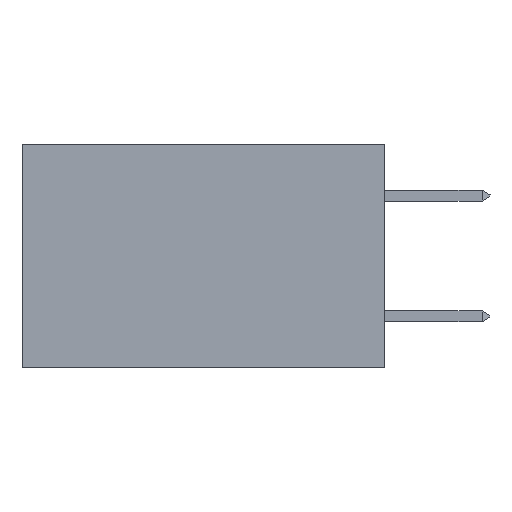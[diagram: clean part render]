
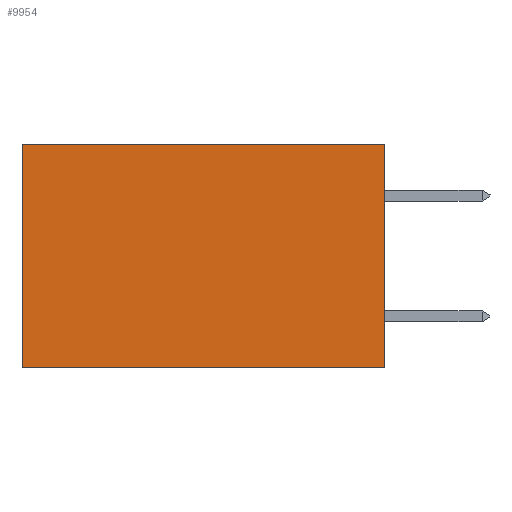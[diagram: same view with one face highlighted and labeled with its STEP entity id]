
A CAD part, left-side view. The second image highlights one B-rep face of the part: STEP entity #9954.
In plain terms, the highlighted planar face has unit normal (-1, 0, 0).
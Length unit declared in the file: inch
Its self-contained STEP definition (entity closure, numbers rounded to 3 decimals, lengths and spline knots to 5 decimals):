
#1040 = VECTOR ( 'NONE', #24002, 39.37008 ) ;
#1258 = LINE ( 'NONE', #24469, #21764 ) ;
#2157 = EDGE_CURVE ( 'NONE', #3082, #12082, #2774, .T. ) ;
#2292 = ORIENTED_EDGE ( 'NONE', *, *, #13835, .F. ) ;
#2747 = FACE_OUTER_BOUND ( 'NONE', #9887, .T. ) ;
#2774 = LINE ( 'NONE', #17856, #18006 ) ;
#3082 = VERTEX_POINT ( 'NONE', #10855 ) ;
#3584 = DIRECTION ( 'NONE',  ( 0., 1., 0. ) ) ;
#6616 = VERTEX_POINT ( 'NONE', #17653 ) ;
#9887 = EDGE_LOOP ( 'NONE', ( #12121, #13611, #2292, #25226 ) ) ;
#9954 = ADVANCED_FACE ( 'NONE', ( #2747 ), #20574, .F. ) ;
#10344 = CARTESIAN_POINT ( 'NONE',  ( 0.2875, 0., -0.37 ) ) ;
#10804 = CARTESIAN_POINT ( 'NONE',  ( 0.2875, 0., 0. ) ) ;
#10855 = CARTESIAN_POINT ( 'NONE',  ( 0.2875, 0., 0. ) ) ;
#12082 = VERTEX_POINT ( 'NONE', #17725 ) ;
#12121 = ORIENTED_EDGE ( 'NONE', *, *, #12992, .T. ) ;
#12232 = LINE ( 'NONE', #17901, #19659 ) ;
#12257 = LINE ( 'NONE', #18019, #1040 ) ;
#12992 = EDGE_CURVE ( 'NONE', #12082, #6616, #12232, .T. ) ;
#13611 = ORIENTED_EDGE ( 'NONE', *, *, #24605, .F. ) ;
#13835 = EDGE_CURVE ( 'NONE', #3082, #18942, #1258, .T. ) ;
#17653 = CARTESIAN_POINT ( 'NONE',  ( 0.2875, 0.6, -0.37 ) ) ;
#17725 = CARTESIAN_POINT ( 'NONE',  ( 0.2875, 0.6, 0. ) ) ;
#17856 = CARTESIAN_POINT ( 'NONE',  ( 0.2875, 0., 0. ) ) ;
#17901 = CARTESIAN_POINT ( 'NONE',  ( 0.2875, 0.6, 0. ) ) ;
#18006 = VECTOR ( 'NONE', #3584, 39.37008 ) ;
#18019 = CARTESIAN_POINT ( 'NONE',  ( 0.2875, 0., -0.37 ) ) ;
#18543 = DIRECTION ( 'NONE',  ( 1., 0., 0. ) ) ;
#18942 = VERTEX_POINT ( 'NONE', #10344 ) ;
#19659 = VECTOR ( 'NONE', #19855, 39.37008 ) ;
#19783 = AXIS2_PLACEMENT_3D ( 'NONE', #10804, #18543, #22570 ) ;
#19855 = DIRECTION ( 'NONE',  ( 0., 0., -1. ) ) ;
#20574 = PLANE ( 'NONE',  #19783 ) ;
#21764 = VECTOR ( 'NONE', #24202, 39.37008 ) ;
#22570 = DIRECTION ( 'NONE',  ( 0., 0., -1. ) ) ;
#24002 = DIRECTION ( 'NONE',  ( 0., 1., 0. ) ) ;
#24202 = DIRECTION ( 'NONE',  ( 0., 0., -1. ) ) ;
#24469 = CARTESIAN_POINT ( 'NONE',  ( 0.2875, 0., 0. ) ) ;
#24605 = EDGE_CURVE ( 'NONE', #18942, #6616, #12257, .T. ) ;
#25226 = ORIENTED_EDGE ( 'NONE', *, *, #2157, .T. ) ;
